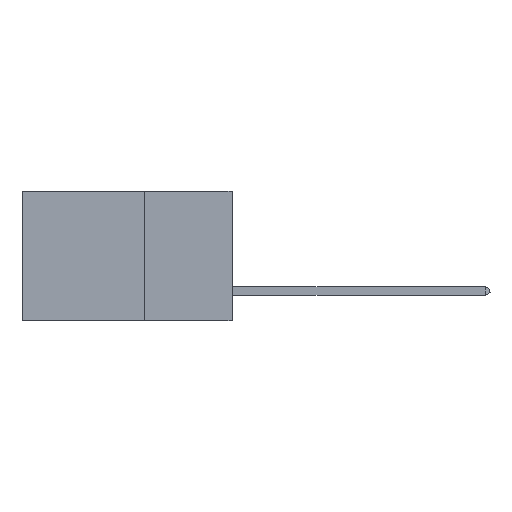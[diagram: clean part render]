
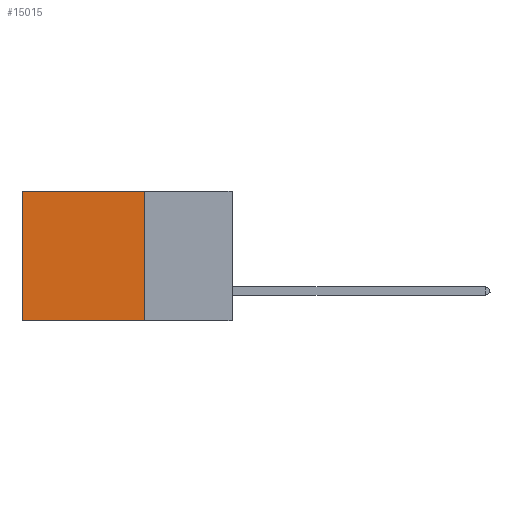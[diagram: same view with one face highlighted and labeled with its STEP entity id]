
A CAD part, left-side view. The second image highlights one B-rep face of the part: STEP entity #15015.
In plain terms, the highlighted planar face has unit normal (-1, 0, 0).
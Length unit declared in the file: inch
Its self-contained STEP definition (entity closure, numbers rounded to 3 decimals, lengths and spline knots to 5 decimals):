
#671 = ORIENTED_EDGE ( 'NONE', *, *, #1413, .F. ) ;
#920 = LINE ( 'NONE', #1161, #30558 ) ;
#1103 = AXIS2_PLACEMENT_3D ( 'NONE', #17317, #24733, #2041 ) ;
#1161 = CARTESIAN_POINT ( 'NONE',  ( 0.2875, 0.6, 0. ) ) ;
#1413 = EDGE_CURVE ( 'NONE', #46595, #19064, #10320, .T. ) ;
#2041 = DIRECTION ( 'NONE',  ( 0., 0., -1. ) ) ;
#3681 = LINE ( 'NONE', #14767, #40414 ) ;
#5373 = ORIENTED_EDGE ( 'NONE', *, *, #12843, .T. ) ;
#6971 = VERTEX_POINT ( 'NONE', #26772 ) ;
#7228 = LINE ( 'NONE', #22283, #22303 ) ;
#10320 = LINE ( 'NONE', #40667, #23208 ) ;
#12071 = ORIENTED_EDGE ( 'NONE', *, *, #44977, .F. ) ;
#12843 = EDGE_CURVE ( 'NONE', #46595, #6971, #3681, .T. ) ;
#12884 = PLANE ( 'NONE',  #1103 ) ;
#14767 = CARTESIAN_POINT ( 'NONE',  ( 0.2875, 0.25, 0. ) ) ;
#15015 = ADVANCED_FACE ( 'NONE', ( #28440 ), #12884, .F. ) ;
#17025 = VERTEX_POINT ( 'NONE', #29193 ) ;
#17317 = CARTESIAN_POINT ( 'NONE',  ( 0.2875, 0.25, 0. ) ) ;
#19064 = VERTEX_POINT ( 'NONE', #24893 ) ;
#22283 = CARTESIAN_POINT ( 'NONE',  ( 0.2875, 0.25, -0.37 ) ) ;
#22303 = VECTOR ( 'NONE', #37323, 39.37008 ) ;
#22671 = DIRECTION ( 'NONE',  ( 0., 0., -1. ) ) ;
#23208 = VECTOR ( 'NONE', #22671, 39.37008 ) ;
#24733 = DIRECTION ( 'NONE',  ( 1., 0., 0. ) ) ;
#24893 = CARTESIAN_POINT ( 'NONE',  ( 0.2875, 0.25, -0.37 ) ) ;
#26772 = CARTESIAN_POINT ( 'NONE',  ( 0.2875, 0.6, 0. ) ) ;
#26837 = DIRECTION ( 'NONE',  ( 0., 0., -1. ) ) ;
#28440 = FACE_OUTER_BOUND ( 'NONE', #37788, .T. ) ;
#29193 = CARTESIAN_POINT ( 'NONE',  ( 0.2875, 0.6, -0.37 ) ) ;
#30558 = VECTOR ( 'NONE', #26837, 39.37008 ) ;
#31851 = EDGE_CURVE ( 'NONE', #6971, #17025, #920, .T. ) ;
#33768 = DIRECTION ( 'NONE',  ( 0., 1., 0. ) ) ;
#37323 = DIRECTION ( 'NONE',  ( 0., 1., 0. ) ) ;
#37788 = EDGE_LOOP ( 'NONE', ( #43780, #12071, #671, #5373 ) ) ;
#40414 = VECTOR ( 'NONE', #33768, 39.37008 ) ;
#40667 = CARTESIAN_POINT ( 'NONE',  ( 0.2875, 0.25, 0. ) ) ;
#43749 = CARTESIAN_POINT ( 'NONE',  ( 0.2875, 0.25, 0. ) ) ;
#43780 = ORIENTED_EDGE ( 'NONE', *, *, #31851, .T. ) ;
#44977 = EDGE_CURVE ( 'NONE', #19064, #17025, #7228, .T. ) ;
#46595 = VERTEX_POINT ( 'NONE', #43749 ) ;
